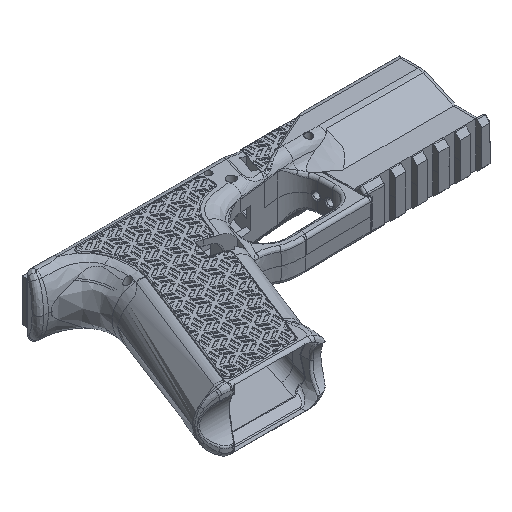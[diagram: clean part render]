
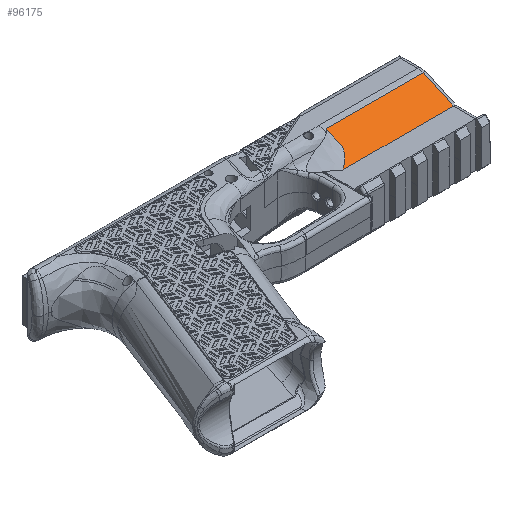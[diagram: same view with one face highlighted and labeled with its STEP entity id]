
A CAD part, isometric view. The second image highlights one B-rep face of the part: STEP entity #96175.
In plain terms, the highlighted planar face has unit normal (0, -0.414, 0.91).
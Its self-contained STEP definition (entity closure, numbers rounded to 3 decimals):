
#2070=B_SPLINE_CURVE_WITH_KNOTS('',3,(#196941,#196942,#196943,#196944,#196945,
#196946,#196947,#196948,#196949,#196950,#196951,#196952,#196953,#196954,
#196955,#196956,#196957,#196958),.UNSPECIFIED.,.F.,.F.,(4,2,2,2,2,2,2,2,
4),(-0.001,0.,0.006,0.02,0.051,
0.116,0.251,0.546,0.933),
 .UNSPECIFIED.);
#5033=PLANE('',#100078);
#10242=FACE_OUTER_BOUND('',#15854,.T.);
#15854=EDGE_LOOP('',(#88680,#88681,#88682,#88683,#88684));
#24822=LINE('',#196960,#33783);
#24824=LINE('',#197002,#33785);
#24826=LINE('',#197008,#33787);
#24827=LINE('',#197009,#33788);
#33783=VECTOR('',#116666,10.);
#33785=VECTOR('',#116670,10.);
#33787=VECTOR('',#116676,10.);
#33788=VECTOR('',#116677,10.);
#46710=VERTEX_POINT('',#196933);
#46711=VERTEX_POINT('',#196940);
#46712=VERTEX_POINT('',#196959);
#46714=VERTEX_POINT('',#197000);
#46716=VERTEX_POINT('',#197007);
#60742=EDGE_CURVE('',#46711,#46710,#2070,.T.);
#60743=EDGE_CURVE('',#46712,#46711,#24822,.T.);
#60746=EDGE_CURVE('',#46710,#46714,#24824,.T.);
#60749=EDGE_CURVE('',#46714,#46716,#24826,.T.);
#60750=EDGE_CURVE('',#46716,#46712,#24827,.T.);
#88680=ORIENTED_EDGE('',*,*,#60749,.T.);
#88681=ORIENTED_EDGE('',*,*,#60750,.T.);
#88682=ORIENTED_EDGE('',*,*,#60743,.T.);
#88683=ORIENTED_EDGE('',*,*,#60742,.T.);
#88684=ORIENTED_EDGE('',*,*,#60746,.T.);
#96175=ADVANCED_FACE('',(#10242),#5033,.F.);
#100078=AXIS2_PLACEMENT_3D('',#197006,#116674,#116675);
#116666=DIRECTION('',(0.,-0.91,-0.414));
#116670=DIRECTION('',(1.,0.,0.));
#116674=DIRECTION('center_axis',(0.,0.414,
-0.91));
#116675=DIRECTION('ref_axis',(0.,-0.91,-0.414));
#116676=DIRECTION('',(0.,0.91,0.414));
#116677=DIRECTION('',(-1.,0.,0.));
#196933=CARTESIAN_POINT('',(118.947,-28.228,7.653));
#196940=CARTESIAN_POINT('',(125.336,-21.215,10.842));
#196941=CARTESIAN_POINT('Ctrl Pts',(125.336,-21.215,
10.842));
#196942=CARTESIAN_POINT('Ctrl Pts',(125.336,-21.219,
10.84));
#196943=CARTESIAN_POINT('Ctrl Pts',(125.335,-21.224,
10.837));
#196944=CARTESIAN_POINT('Ctrl Pts',(125.334,-21.247,
10.827));
#196945=CARTESIAN_POINT('Ctrl Pts',(125.333,-21.269,
10.817));
#196946=CARTESIAN_POINT('Ctrl Pts',(125.326,-21.334,10.788));
#196947=CARTESIAN_POINT('Ctrl Pts',(125.319,-21.38,
10.767));
#196948=CARTESIAN_POINT('Ctrl Pts',(125.294,-21.522,10.702));
#196949=CARTESIAN_POINT('Ctrl Pts',(125.27,-21.623,
10.656));
#196950=CARTESIAN_POINT('Ctrl Pts',(125.187,-21.925,10.519));
#196951=CARTESIAN_POINT('Ctrl Pts',(125.111,-22.131,
10.425));
#196952=CARTESIAN_POINT('Ctrl Pts',(124.851,-22.744,
10.146));
#196953=CARTESIAN_POINT('Ctrl Pts',(124.622,-23.152,9.961));
#196954=CARTESIAN_POINT('Ctrl Pts',(123.817,-24.371,
9.407));
#196955=CARTESIAN_POINT('Ctrl Pts',(123.112,-25.147,
9.054));
#196956=CARTESIAN_POINT('Ctrl Pts',(121.333,-26.748,
8.326));
#196957=CARTESIAN_POINT('Ctrl Pts',(120.181,-27.542,
7.965));
#196958=CARTESIAN_POINT('Ctrl Pts',(118.947,-28.228,
7.653));
#196959=CARTESIAN_POINT('',(125.336,-14.119,14.068));
#196960=CARTESIAN_POINT('',(125.336,-31.736,6.058));
#197000=CARTESIAN_POINT('',(170.336,-28.228,7.653));
#197002=CARTESIAN_POINT('',(163.653,-28.228,7.653));
#197006=CARTESIAN_POINT('Origin',(172.336,-14.119,14.068));
#197007=CARTESIAN_POINT('',(170.336,-14.119,14.068));
#197008=CARTESIAN_POINT('',(170.336,-27.664,7.91));
#197009=CARTESIAN_POINT('',(124.336,-14.119,14.068));
